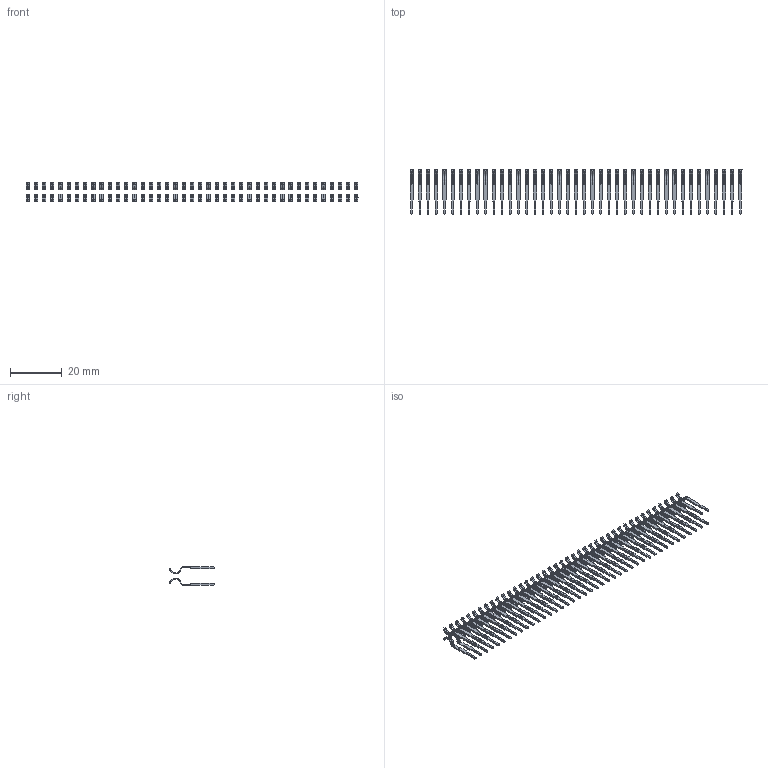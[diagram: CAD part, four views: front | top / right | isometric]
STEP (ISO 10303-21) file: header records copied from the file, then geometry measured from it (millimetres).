
FILE_DESCRIPTION (( 'STEP AP203' ), '1' );
FILE_NAME ('346-082-521-812.STEP', '2018-08-29T09:06:14', ( '' ), ( '' ), 'SwSTEP 2.0', 'SolidWorks 2016', '' );
FILE_SCHEMA (( 'CONFIG_CONTROL_DESIGN' ));
Length unit declared in the file: inch
Products named in the file (3): 346 Part_0.170 Offset - Side Mount; 345-292-001_345-293-121; 346-082-521-812
Assembly tree (83 placements, depth 2):
  346-082-521-812
    346 Part_0.170 Offset - Side Mount
    345-292-001_345-293-121  x82
Bounding box: 128.27 x 17.14 x 6.99 mm (x, y, z)
Volume: 704.4 mm3; surface area: 4998.4 mm2
Topology: 82 solids, 82 shells, 3772 faces, 10988 edges, 7216 vertices
Faces by surface type: plane 2460, cylinder 1312
Entity records: 27045 total; most frequent: CARTESIAN_POINT 4460, ORIENTED_EDGE 4394, DIRECTION 3981, EDGE_CURVE 2197, LINE 1901, VECTOR 1901, VERTEX_POINT 1462, AXIS2_PLACEMENT_3D 1040
